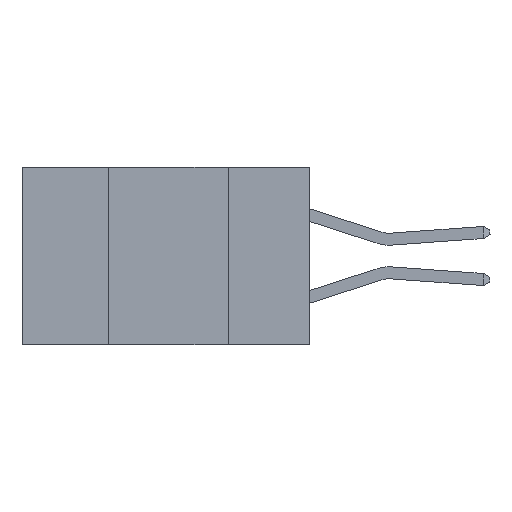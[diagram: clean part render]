
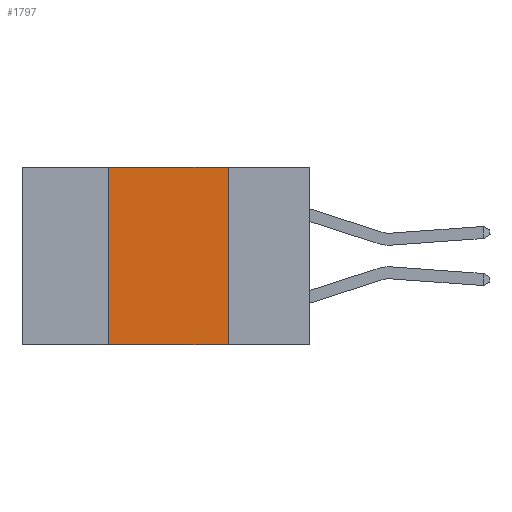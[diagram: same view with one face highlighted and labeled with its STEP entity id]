
A CAD part, left-side view. The second image highlights one B-rep face of the part: STEP entity #1797.
In plain terms, the highlighted planar face has unit normal (-1, 0, 0).
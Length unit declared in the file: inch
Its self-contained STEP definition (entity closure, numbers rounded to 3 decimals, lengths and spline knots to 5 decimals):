
#662 = CARTESIAN_POINT ( 'NONE',  ( 0., 0.42, -0.37 ) ) ;
#848 = ORIENTED_EDGE ( 'NONE', *, *, #5680, .F. ) ;
#1077 = VERTEX_POINT ( 'NONE', #16300 ) ;
#1797 = ADVANCED_FACE ( 'NONE', ( #13795 ), #15257, .F. ) ;
#1964 = DIRECTION ( 'NONE',  ( 1., 0., 0. ) ) ;
#2201 = VERTEX_POINT ( 'NONE', #8061 ) ;
#3328 = EDGE_CURVE ( 'NONE', #5557, #13719, #18444, .T. ) ;
#3509 = CARTESIAN_POINT ( 'NONE',  ( 0., 0.6, 0. ) ) ;
#5067 = CARTESIAN_POINT ( 'NONE',  ( 0., 0.6, -0.37 ) ) ;
#5557 = VERTEX_POINT ( 'NONE', #7296 ) ;
#5680 = EDGE_CURVE ( 'NONE', #2201, #1077, #8653, .T. ) ;
#6341 = VECTOR ( 'NONE', #15904, 39.37008 ) ;
#6386 = LINE ( 'NONE', #12120, #15914 ) ;
#6526 = DIRECTION ( 'NONE',  ( 0., 0., -1. ) ) ;
#6598 = DIRECTION ( 'NONE',  ( 0., 0., 1. ) ) ;
#7296 = CARTESIAN_POINT ( 'NONE',  ( 0., 0.42, -0.37 ) ) ;
#7484 = CARTESIAN_POINT ( 'NONE',  ( 0., 0.17, -0.37 ) ) ;
#8061 = CARTESIAN_POINT ( 'NONE',  ( 0., 0.17, 0. ) ) ;
#8533 = EDGE_CURVE ( 'NONE', #13719, #2201, #6386, .T. ) ;
#8653 = LINE ( 'NONE', #7484, #6341 ) ;
#9647 = LINE ( 'NONE', #5067, #11789 ) ;
#11469 = CARTESIAN_POINT ( 'NONE',  ( 0., 0.42, 0. ) ) ;
#11789 = VECTOR ( 'NONE', #17010, 39.37008 ) ;
#12120 = CARTESIAN_POINT ( 'NONE',  ( 0., 0.6, 0. ) ) ;
#13120 = VECTOR ( 'NONE', #6598, 39.37008 ) ;
#13392 = ORIENTED_EDGE ( 'NONE', *, *, #3328, .F. ) ;
#13595 = ORIENTED_EDGE ( 'NONE', *, *, #8533, .F. ) ;
#13719 = VERTEX_POINT ( 'NONE', #11469 ) ;
#13795 = FACE_OUTER_BOUND ( 'NONE', #18056, .T. ) ;
#14012 = AXIS2_PLACEMENT_3D ( 'NONE', #3509, #1964, #6526 ) ;
#15257 = PLANE ( 'NONE',  #14012 ) ;
#15904 = DIRECTION ( 'NONE',  ( 0., 0., -1. ) ) ;
#15914 = VECTOR ( 'NONE', #18034, 39.37008 ) ;
#16300 = CARTESIAN_POINT ( 'NONE',  ( 0., 0.17, -0.37 ) ) ;
#17010 = DIRECTION ( 'NONE',  ( 0., -1., 0. ) ) ;
#18034 = DIRECTION ( 'NONE',  ( 0., -1., 0. ) ) ;
#18056 = EDGE_LOOP ( 'NONE', ( #848, #13595, #13392, #18848 ) ) ;
#18444 = LINE ( 'NONE', #662, #13120 ) ;
#18725 = EDGE_CURVE ( 'NONE', #5557, #1077, #9647, .T. ) ;
#18848 = ORIENTED_EDGE ( 'NONE', *, *, #18725, .T. ) ;
